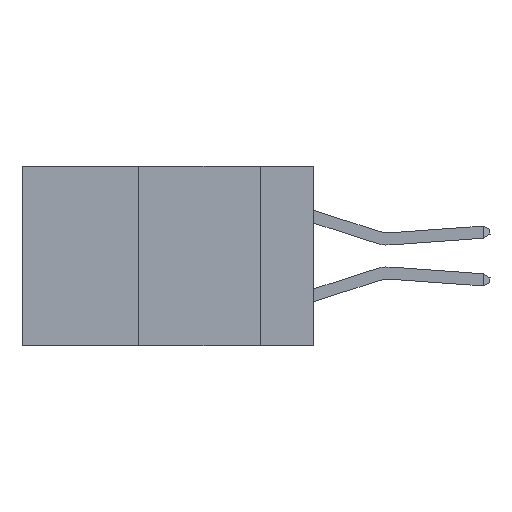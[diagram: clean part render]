
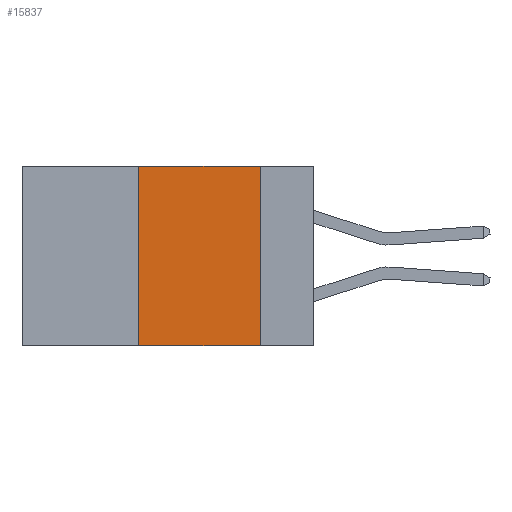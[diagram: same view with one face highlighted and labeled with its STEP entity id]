
A CAD part, left-side view. The second image highlights one B-rep face of the part: STEP entity #15837.
In plain terms, the highlighted planar face has unit normal (-1, 0, 0).
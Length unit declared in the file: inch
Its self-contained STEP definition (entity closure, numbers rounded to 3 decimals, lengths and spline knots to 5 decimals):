
#1400 = DIRECTION ( 'NONE',  ( 0., 0., -1. ) ) ;
#1772 = ORIENTED_EDGE ( 'NONE', *, *, #2601, .F. ) ;
#2601 = EDGE_CURVE ( 'NONE', #18202, #13538, #12492, .T. ) ;
#2903 = VECTOR ( 'NONE', #8939, 39.37008 ) ;
#2922 = CARTESIAN_POINT ( 'NONE',  ( 0., 0.11, 0. ) ) ;
#3416 = VERTEX_POINT ( 'NONE', #31492 ) ;
#4303 = DIRECTION ( 'NONE',  ( 0., 0., 1. ) ) ;
#8939 = DIRECTION ( 'NONE',  ( 0., -1., 0. ) ) ;
#9411 = LINE ( 'NONE', #12122, #21460 ) ;
#9845 = VECTOR ( 'NONE', #23502, 39.37008 ) ;
#11603 = DIRECTION ( 'NONE',  ( 1., 0., 0. ) ) ;
#12122 = CARTESIAN_POINT ( 'NONE',  ( 0., 0.36, 0. ) ) ;
#12492 = LINE ( 'NONE', #13684, #25294 ) ;
#13145 = VERTEX_POINT ( 'NONE', #20914 ) ;
#13538 = VERTEX_POINT ( 'NONE', #29773 ) ;
#13684 = CARTESIAN_POINT ( 'NONE',  ( 0., 0.11, 0. ) ) ;
#15837 = ADVANCED_FACE ( 'NONE', ( #18627 ), #19268, .F. ) ;
#17231 = ORIENTED_EDGE ( 'NONE', *, *, #27852, .F. ) ;
#17501 = LINE ( 'NONE', #20961, #9845 ) ;
#18202 = VERTEX_POINT ( 'NONE', #2922 ) ;
#18627 = FACE_OUTER_BOUND ( 'NONE', #32152, .T. ) ;
#19268 = PLANE ( 'NONE',  #21506 ) ;
#20914 = CARTESIAN_POINT ( 'NONE',  ( 0., 0.36, 0. ) ) ;
#20961 = CARTESIAN_POINT ( 'NONE',  ( 0., 0.6, 0. ) ) ;
#21114 = EDGE_CURVE ( 'NONE', #3416, #13538, #23516, .T. ) ;
#21460 = VECTOR ( 'NONE', #4303, 39.37008 ) ;
#21506 = AXIS2_PLACEMENT_3D ( 'NONE', #26915, #11603, #29403 ) ;
#21537 = EDGE_CURVE ( 'NONE', #13145, #18202, #17501, .T. ) ;
#21873 = CARTESIAN_POINT ( 'NONE',  ( 0., 0.6, -0.37 ) ) ;
#23502 = DIRECTION ( 'NONE',  ( 0., -1., 0. ) ) ;
#23516 = LINE ( 'NONE', #21873, #2903 ) ;
#25294 = VECTOR ( 'NONE', #1400, 39.37008 ) ;
#26001 = ORIENTED_EDGE ( 'NONE', *, *, #21537, .F. ) ;
#26367 = ORIENTED_EDGE ( 'NONE', *, *, #21114, .T. ) ;
#26915 = CARTESIAN_POINT ( 'NONE',  ( 0., 0.6, 0. ) ) ;
#27852 = EDGE_CURVE ( 'NONE', #3416, #13145, #9411, .T. ) ;
#29403 = DIRECTION ( 'NONE',  ( 0., 0., -1. ) ) ;
#29773 = CARTESIAN_POINT ( 'NONE',  ( 0., 0.11, -0.37 ) ) ;
#31492 = CARTESIAN_POINT ( 'NONE',  ( 0., 0.36, -0.37 ) ) ;
#32152 = EDGE_LOOP ( 'NONE', ( #1772, #26001, #17231, #26367 ) ) ;
